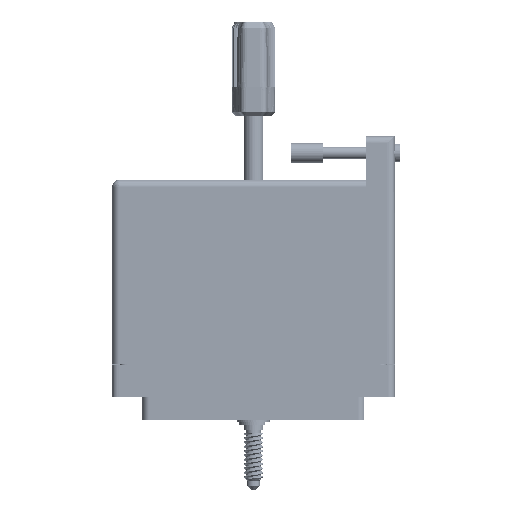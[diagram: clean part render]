
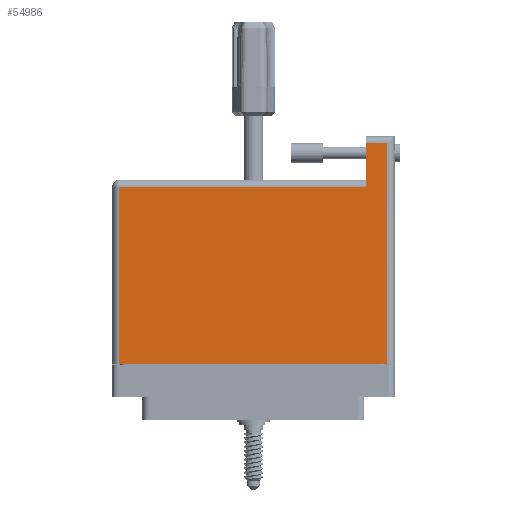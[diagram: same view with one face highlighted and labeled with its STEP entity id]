
A CAD part, front view. The second image highlights one B-rep face of the part: STEP entity #54986.
In plain terms, the highlighted face is planar.
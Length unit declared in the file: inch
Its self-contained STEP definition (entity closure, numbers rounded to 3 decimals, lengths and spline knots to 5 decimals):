
#2445 = VECTOR ( 'NONE', #36619, 39.37008 ) ;
#2614 = ORIENTED_EDGE ( 'NONE', *, *, #73294, .T. ) ;
#3309 = VERTEX_POINT ( 'NONE', #41986 ) ;
#6454 = AXIS2_PLACEMENT_3D ( 'NONE', #58560, #18256, #44801 ) ;
#8754 = DIRECTION ( 'NONE',  ( -1., 0., 0. ) ) ;
#10406 = CARTESIAN_POINT ( 'NONE',  ( -1.359, 2.025, 0.617 ) ) ;
#12362 = EDGE_CURVE ( 'NONE', #59075, #3309, #86009, .T. ) ;
#13901 = VECTOR ( 'NONE', #8754, 39.37008 ) ;
#14166 = ORIENTED_EDGE ( 'NONE', *, *, #12362, .T. ) ;
#18256 = DIRECTION ( 'NONE',  ( 0., 0., -1. ) ) ;
#18499 = DIRECTION ( 'NONE',  ( 0., -1., 0. ) ) ;
#21306 = EDGE_CURVE ( 'NONE', #41326, #54827, #30166, .T. ) ;
#21492 = CARTESIAN_POINT ( 'NONE',  ( 1.079, 1.605, 0.617 ) ) ;
#21620 = CARTESIAN_POINT ( 'NONE',  ( -1.359, 1.605, 0.617 ) ) ;
#22456 = CARTESIAN_POINT ( 'NONE',  ( 1.289, 2.025, 0.617 ) ) ;
#23934 = VECTOR ( 'NONE', #57389, 39.37008 ) ;
#24029 = CARTESIAN_POINT ( 'NONE',  ( -1.359, -0.1, 0.617 ) ) ;
#24870 = VECTOR ( 'NONE', #63297, 39.37008 ) ;
#25391 = EDGE_CURVE ( 'NONE', #28846, #41326, #34431, .T. ) ;
#26811 = DIRECTION ( 'NONE',  ( 0., -1., 0. ) ) ;
#28029 = CARTESIAN_POINT ( 'NONE',  ( 1.079, 2.025, 0.617 ) ) ;
#28846 = VERTEX_POINT ( 'NONE', #22456 ) ;
#30166 = LINE ( 'NONE', #52273, #85569 ) ;
#32173 = LINE ( 'NONE', #37607, #24870 ) ;
#34431 = LINE ( 'NONE', #10406, #23934 ) ;
#35574 = ORIENTED_EDGE ( 'NONE', *, *, #66201, .T. ) ;
#36619 = DIRECTION ( 'NONE',  ( 1., 0., 0. ) ) ;
#37313 = PLANE ( 'NONE',  #6454 ) ;
#37482 = EDGE_CURVE ( 'NONE', #54827, #44408, #57839, .T. ) ;
#37607 = CARTESIAN_POINT ( 'NONE',  ( 1.289, 2.095, 0.617 ) ) ;
#41326 = VERTEX_POINT ( 'NONE', #28029 ) ;
#41986 = CARTESIAN_POINT ( 'NONE',  ( 1.289, -0.1, 0.617 ) ) ;
#44408 = VERTEX_POINT ( 'NONE', #81039 ) ;
#44801 = DIRECTION ( 'NONE',  ( -1., 0., 0. ) ) ;
#46404 = ORIENTED_EDGE ( 'NONE', *, *, #21306, .T. ) ;
#48391 = FACE_OUTER_BOUND ( 'NONE', #80243, .T. ) ;
#52273 = CARTESIAN_POINT ( 'NONE',  ( 1.079, 2.095, 0.617 ) ) ;
#54723 = LINE ( 'NONE', #73550, #85217 ) ;
#54827 = VERTEX_POINT ( 'NONE', #21492 ) ;
#54986 = ADVANCED_FACE ( 'NONE', ( #48391 ), #37313, .F. ) ;
#57389 = DIRECTION ( 'NONE',  ( -1., 0., 0. ) ) ;
#57839 = LINE ( 'NONE', #21620, #13901 ) ;
#58560 = CARTESIAN_POINT ( 'NONE',  ( -1.359, 1.675, 0.617 ) ) ;
#59075 = VERTEX_POINT ( 'NONE', #80250 ) ;
#63297 = DIRECTION ( 'NONE',  ( 0., 1., 0. ) ) ;
#66201 = EDGE_CURVE ( 'NONE', #44408, #59075, #54723, .T. ) ;
#73294 = EDGE_CURVE ( 'NONE', #3309, #28846, #32173, .T. ) ;
#73550 = CARTESIAN_POINT ( 'NONE',  ( -1.289, -0.1, 0.617 ) ) ;
#80243 = EDGE_LOOP ( 'NONE', ( #80448, #35574, #14166, #2614, #81948, #46404 ) ) ;
#80250 = CARTESIAN_POINT ( 'NONE',  ( -1.289, -0.1, 0.617 ) ) ;
#80448 = ORIENTED_EDGE ( 'NONE', *, *, #37482, .T. ) ;
#81039 = CARTESIAN_POINT ( 'NONE',  ( -1.289, 1.605, 0.617 ) ) ;
#81948 = ORIENTED_EDGE ( 'NONE', *, *, #25391, .T. ) ;
#85217 = VECTOR ( 'NONE', #26811, 39.37008 ) ;
#85569 = VECTOR ( 'NONE', #18499, 39.37008 ) ;
#86009 = LINE ( 'NONE', #24029, #2445 ) ;
